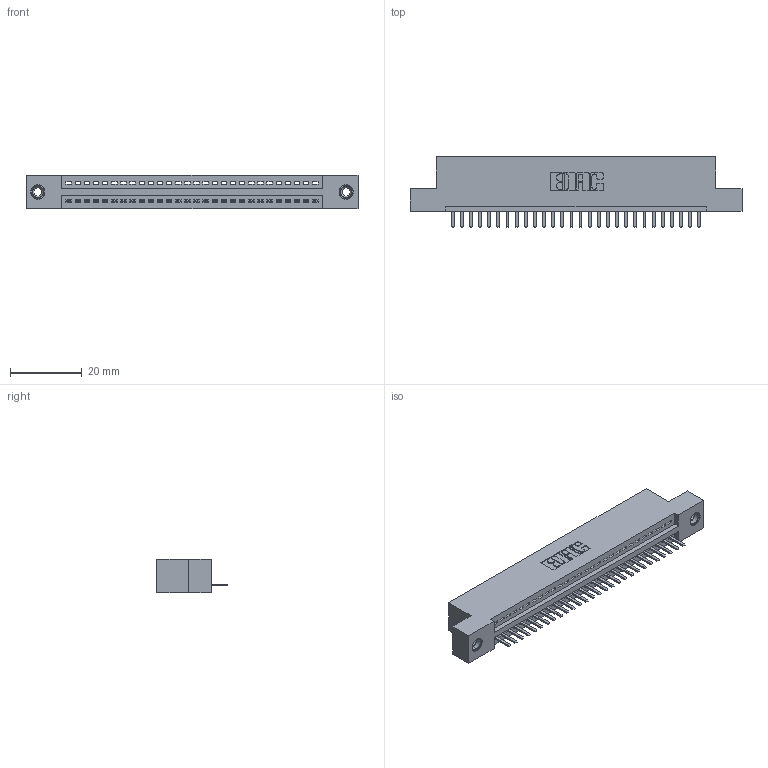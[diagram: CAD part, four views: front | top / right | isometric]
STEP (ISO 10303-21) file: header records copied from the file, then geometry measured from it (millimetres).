
FILE_DESCRIPTION (( 'STEP AP203' ), '1' );
FILE_NAME ('395-028-520-108.STEP', '2019-10-19T03:11:30', ( '' ), ( '' ), 'SwSTEP 2.0', 'SolidWorks 2016', '' );
FILE_SCHEMA (( 'CONFIG_CONTROL_DESIGN' ));
Length unit declared in the file: inch
Products named in the file (4): 345-250-001_345-250-003-102; 345-292-001_345-293-120; 395-028-520-108; 345 Part_Flush Mounting Lugs - 0.156 Dia-TI
Assembly tree (31 placements, depth 2):
  395-028-520-108
    345 Part_Flush Mounting Lugs - 0.156 Dia-TI
    345-292-001_345-293-120  x28
    345-250-001_345-250-003-102  x2
Bounding box: 92.33 x 19.68 x 9.4 mm (x, y, z)
Volume: 8567.8 mm3; surface area: 10951.2 mm2
Topology: 31 solids, 31 shells, 1922 faces, 5629 edges, 3670 vertices
Faces by surface type: plane 1288, cylinder 618, cone 12, torus 4
Entity records: 24258 total; most frequent: CARTESIAN_POINT 4195, ORIENTED_EDGE 4138, DIRECTION 3699, EDGE_CURVE 2069, LINE 1801, VECTOR 1801, VERTEX_POINT 1372, AXIS2_PLACEMENT_3D 949
